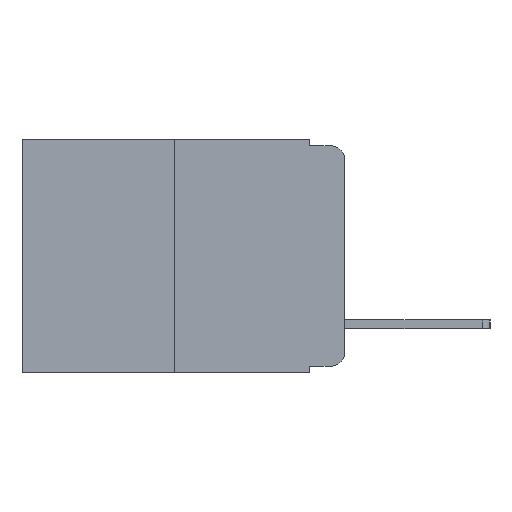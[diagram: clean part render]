
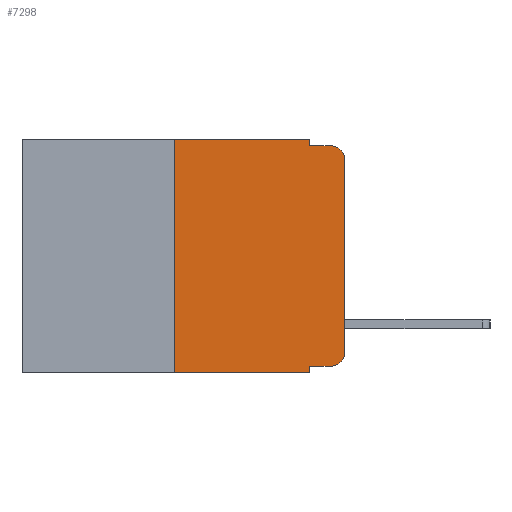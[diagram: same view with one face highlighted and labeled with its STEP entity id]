
A CAD part, left-side view. The second image highlights one B-rep face of the part: STEP entity #7298.
In plain terms, the highlighted planar face has unit normal (-1, 0, 0).
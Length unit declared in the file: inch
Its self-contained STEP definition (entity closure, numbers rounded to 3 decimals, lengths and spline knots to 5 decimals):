
#94 = DIRECTION ( 'NONE',  ( 0., 0., -1. ) ) ;
#390 = FACE_OUTER_BOUND ( 'NONE', #4216, .T. ) ;
#506 = VERTEX_POINT ( 'NONE', #9875 ) ;
#572 = CARTESIAN_POINT ( 'NONE',  ( 0., 0.25, 0. ) ) ;
#655 = CARTESIAN_POINT ( 'NONE',  ( 0., 0.051, -0.343 ) ) ;
#938 = ORIENTED_EDGE ( 'NONE', *, *, #4084, .T. ) ;
#1375 = VECTOR ( 'NONE', #13169, 39.37008 ) ;
#1439 = AXIS2_PLACEMENT_3D ( 'NONE', #12808, #6557, #94 ) ;
#1564 = AXIS2_PLACEMENT_3D ( 'NONE', #5291, #12646, #6383 ) ;
#1663 = DIRECTION ( 'NONE',  ( 0., 0., 1. ) ) ;
#2097 = DIRECTION ( 'NONE',  ( 0., 0., -1. ) ) ;
#2138 = VECTOR ( 'NONE', #7220, 39.37008 ) ;
#2146 = VECTOR ( 'NONE', #8117, 39.37008 ) ;
#2242 = ORIENTED_EDGE ( 'NONE', *, *, #10072, .T. ) ;
#2255 = LINE ( 'NONE', #6747, #7686 ) ;
#2388 = CARTESIAN_POINT ( 'NONE',  ( 0., 0., -0.313 ) ) ;
#2735 = VERTEX_POINT ( 'NONE', #655 ) ;
#2899 = VERTEX_POINT ( 'NONE', #3954 ) ;
#2983 = ORIENTED_EDGE ( 'NONE', *, *, #6141, .T. ) ;
#3345 = CARTESIAN_POINT ( 'NONE',  ( 0., 0., 0. ) ) ;
#3514 = ORIENTED_EDGE ( 'NONE', *, *, #5152, .F. ) ;
#3551 = ORIENTED_EDGE ( 'NONE', *, *, #9140, .F. ) ;
#3639 = DIRECTION ( 'NONE',  ( 0., -1., 0. ) ) ;
#3954 = CARTESIAN_POINT ( 'NONE',  ( 0., 0.02, -0.333 ) ) ;
#4084 = EDGE_CURVE ( 'NONE', #12366, #6902, #9323, .T. ) ;
#4216 = EDGE_LOOP ( 'NONE', ( #2983, #938, #4348, #3514, #3551, #9273, #6085, #11057, #7535, #2242 ) ) ;
#4296 = CARTESIAN_POINT ( 'NONE',  ( 0., 0.051, -0.333 ) ) ;
#4348 = ORIENTED_EDGE ( 'NONE', *, *, #11631, .F. ) ;
#4628 = LINE ( 'NONE', #8305, #9657 ) ;
#5152 = EDGE_CURVE ( 'NONE', #7771, #506, #13062, .T. ) ;
#5291 = CARTESIAN_POINT ( 'NONE',  ( 0., 0.02, -0.03 ) ) ;
#5380 = AXIS2_PLACEMENT_3D ( 'NONE', #7495, #8562, #2097 ) ;
#5513 = DIRECTION ( 'NONE',  ( 0., 0., 1. ) ) ;
#5715 = EDGE_CURVE ( 'NONE', #8420, #8274, #5834, .T. ) ;
#5823 = VECTOR ( 'NONE', #5513, 39.37008 ) ;
#5834 = LINE ( 'NONE', #572, #8390 ) ;
#5836 = CARTESIAN_POINT ( 'NONE',  ( 0., 0.051, 0. ) ) ;
#6085 = ORIENTED_EDGE ( 'NONE', *, *, #13081, .T. ) ;
#6141 = EDGE_CURVE ( 'NONE', #6820, #12366, #8706, .T. ) ;
#6237 = CIRCLE ( 'NONE', #1439, 0.02 ) ;
#6383 = DIRECTION ( 'NONE',  ( 0., 0., -1. ) ) ;
#6529 = EDGE_CURVE ( 'NONE', #7341, #2899, #4628, .T. ) ;
#6557 = DIRECTION ( 'NONE',  ( -1., 0., 0. ) ) ;
#6747 = CARTESIAN_POINT ( 'NONE',  ( 0., 0.473, -0.343 ) ) ;
#6784 = LINE ( 'NONE', #8982, #12000 ) ;
#6820 = VERTEX_POINT ( 'NONE', #2388 ) ;
#6902 = VERTEX_POINT ( 'NONE', #10004 ) ;
#7220 = DIRECTION ( 'NONE',  ( 0., -1., 0. ) ) ;
#7298 = ADVANCED_FACE ( 'NONE', ( #390 ), #13688, .F. ) ;
#7341 = VERTEX_POINT ( 'NONE', #4296 ) ;
#7427 = CARTESIAN_POINT ( 'NONE',  ( 0., 0.051, 0. ) ) ;
#7495 = CARTESIAN_POINT ( 'NONE',  ( 0., 0.473, 0. ) ) ;
#7535 = ORIENTED_EDGE ( 'NONE', *, *, #6529, .T. ) ;
#7686 = VECTOR ( 'NONE', #10947, 39.37008 ) ;
#7771 = VERTEX_POINT ( 'NONE', #7427 ) ;
#8040 = CARTESIAN_POINT ( 'NONE',  ( 0., 0.051, 0. ) ) ;
#8082 = EDGE_CURVE ( 'NONE', #7341, #2735, #9604, .T. ) ;
#8117 = DIRECTION ( 'NONE',  ( 0., 0., -1. ) ) ;
#8274 = VERTEX_POINT ( 'NONE', #9299 ) ;
#8305 = CARTESIAN_POINT ( 'NONE',  ( 0., 0.051, -0.333 ) ) ;
#8390 = VECTOR ( 'NONE', #1663, 39.37008 ) ;
#8420 = VERTEX_POINT ( 'NONE', #9521 ) ;
#8562 = DIRECTION ( 'NONE',  ( 1., 0., 0. ) ) ;
#8706 = LINE ( 'NONE', #3345, #5823 ) ;
#8982 = CARTESIAN_POINT ( 'NONE',  ( 0., 0.473, 0. ) ) ;
#9140 = EDGE_CURVE ( 'NONE', #8274, #7771, #6784, .T. ) ;
#9273 = ORIENTED_EDGE ( 'NONE', *, *, #5715, .F. ) ;
#9299 = CARTESIAN_POINT ( 'NONE',  ( 0., 0.25, 0. ) ) ;
#9323 = CIRCLE ( 'NONE', #1564, 0.02 ) ;
#9389 = DIRECTION ( 'NONE',  ( 0., -1., 0. ) ) ;
#9521 = CARTESIAN_POINT ( 'NONE',  ( 0., 0.25, -0.343 ) ) ;
#9604 = LINE ( 'NONE', #5836, #1375 ) ;
#9657 = VECTOR ( 'NONE', #9389, 39.37008 ) ;
#9875 = CARTESIAN_POINT ( 'NONE',  ( 0., 0.051, -0.01 ) ) ;
#10004 = CARTESIAN_POINT ( 'NONE',  ( 0., 0.02, -0.01 ) ) ;
#10072 = EDGE_CURVE ( 'NONE', #2899, #6820, #6237, .T. ) ;
#10524 = CARTESIAN_POINT ( 'NONE',  ( 0., 0., -0.03 ) ) ;
#10947 = DIRECTION ( 'NONE',  ( 0., -1., 0. ) ) ;
#11057 = ORIENTED_EDGE ( 'NONE', *, *, #8082, .F. ) ;
#11631 = EDGE_CURVE ( 'NONE', #506, #6902, #13378, .T. ) ;
#12000 = VECTOR ( 'NONE', #3639, 39.37008 ) ;
#12366 = VERTEX_POINT ( 'NONE', #10524 ) ;
#12392 = CARTESIAN_POINT ( 'NONE',  ( 0., 0.051, -0.01 ) ) ;
#12646 = DIRECTION ( 'NONE',  ( -1., 0., 0. ) ) ;
#12808 = CARTESIAN_POINT ( 'NONE',  ( 0., 0.02, -0.313 ) ) ;
#13062 = LINE ( 'NONE', #8040, #2146 ) ;
#13081 = EDGE_CURVE ( 'NONE', #8420, #2735, #2255, .T. ) ;
#13169 = DIRECTION ( 'NONE',  ( 0., 0., -1. ) ) ;
#13378 = LINE ( 'NONE', #12392, #2138 ) ;
#13688 = PLANE ( 'NONE',  #5380 ) ;
